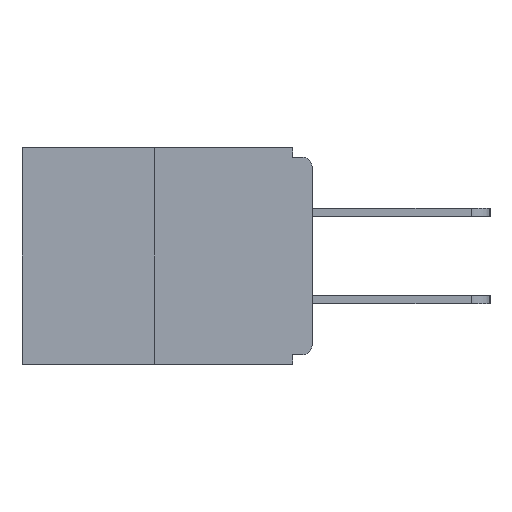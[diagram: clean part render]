
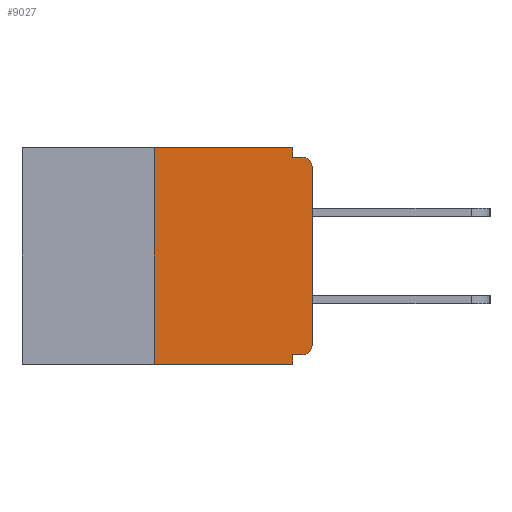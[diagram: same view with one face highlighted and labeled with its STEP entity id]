
A CAD part, left-side view. The second image highlights one B-rep face of the part: STEP entity #9027.
In plain terms, the highlighted planar face has unit normal (-1, 0, 0).
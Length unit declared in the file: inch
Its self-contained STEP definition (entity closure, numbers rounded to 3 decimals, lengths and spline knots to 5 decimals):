
#261 = CARTESIAN_POINT ( 'NONE',  ( 0., 0., -0.313 ) ) ;
#437 = ORIENTED_EDGE ( 'NONE', *, *, #20710, .F. ) ;
#1128 = DIRECTION ( 'NONE',  ( 0., 0., -1. ) ) ;
#1268 = DIRECTION ( 'NONE',  ( 0., 0., 1. ) ) ;
#1305 = CARTESIAN_POINT ( 'NONE',  ( 0., 0.031, -0.015 ) ) ;
#1524 = CARTESIAN_POINT ( 'NONE',  ( 0., 0., 0. ) ) ;
#2679 = LINE ( 'NONE', #7748, #10173 ) ;
#2927 = AXIS2_PLACEMENT_3D ( 'NONE', #16775, #23106, #1128 ) ;
#3027 = LINE ( 'NONE', #24769, #15173 ) ;
#3194 = ORIENTED_EDGE ( 'NONE', *, *, #22684, .T. ) ;
#3237 = DIRECTION ( 'NONE',  ( 0., -1., 0. ) ) ;
#3621 = CARTESIAN_POINT ( 'NONE',  ( 0., 0.031, 0. ) ) ;
#3947 = FACE_OUTER_BOUND ( 'NONE', #13196, .T. ) ;
#4283 = LINE ( 'NONE', #8755, #5694 ) ;
#4379 = AXIS2_PLACEMENT_3D ( 'NONE', #14721, #16600, #27711 ) ;
#4413 = EDGE_CURVE ( 'NONE', #26458, #11795, #27263, .T. ) ;
#4925 = CARTESIAN_POINT ( 'NONE',  ( 0., 0., -0.03 ) ) ;
#5112 = CARTESIAN_POINT ( 'NONE',  ( 0., 0.031, -0.328 ) ) ;
#5694 = VECTOR ( 'NONE', #12999, 39.37008 ) ;
#6394 = ORIENTED_EDGE ( 'NONE', *, *, #4413, .T. ) ;
#6710 = EDGE_CURVE ( 'NONE', #12282, #9344, #3027, .T. ) ;
#7748 = CARTESIAN_POINT ( 'NONE',  ( 0., 0.031, -0.343 ) ) ;
#8276 = CARTESIAN_POINT ( 'NONE',  ( 0., 0.015, -0.328 ) ) ;
#8527 = DIRECTION ( 'NONE',  ( 0., 0., -1. ) ) ;
#8755 = CARTESIAN_POINT ( 'NONE',  ( 0., 0., -0.328 ) ) ;
#9027 = ADVANCED_FACE ( 'NONE', ( #3947 ), #27689, .F. ) ;
#9151 = CARTESIAN_POINT ( 'NONE',  ( 0., 0.25, -0.343 ) ) ;
#9344 = VERTEX_POINT ( 'NONE', #3621 ) ;
#9543 = DIRECTION ( 'NONE',  ( 0., -1., 0. ) ) ;
#10173 = VECTOR ( 'NONE', #20523, 39.37008 ) ;
#10186 = VERTEX_POINT ( 'NONE', #8276 ) ;
#10757 = DIRECTION ( 'NONE',  ( 0., 0., -1. ) ) ;
#10829 = VERTEX_POINT ( 'NONE', #261 ) ;
#10928 = EDGE_CURVE ( 'NONE', #23420, #19906, #15781, .T. ) ;
#11022 = CARTESIAN_POINT ( 'NONE',  ( 0., 0.015, -0.015 ) ) ;
#11795 = VERTEX_POINT ( 'NONE', #24815 ) ;
#11816 = ORIENTED_EDGE ( 'NONE', *, *, #22833, .T. ) ;
#11881 = CARTESIAN_POINT ( 'NONE',  ( 0., 0., -0.015 ) ) ;
#12282 = VERTEX_POINT ( 'NONE', #23031 ) ;
#12361 = ORIENTED_EDGE ( 'NONE', *, *, #6710, .F. ) ;
#12999 = DIRECTION ( 'NONE',  ( 0., 1., 0. ) ) ;
#13196 = EDGE_LOOP ( 'NONE', ( #12361, #14241, #6394, #20639, #13666, #11816, #3194, #20376, #25923, #437 ) ) ;
#13666 = ORIENTED_EDGE ( 'NONE', *, *, #19417, .F. ) ;
#14241 = ORIENTED_EDGE ( 'NONE', *, *, #21060, .F. ) ;
#14721 = CARTESIAN_POINT ( 'NONE',  ( 0., 0.015, -0.313 ) ) ;
#15173 = VECTOR ( 'NONE', #9543, 39.37008 ) ;
#15293 = VECTOR ( 'NONE', #20258, 39.37008 ) ;
#15540 = CARTESIAN_POINT ( 'NONE',  ( 0., 0.46, 0. ) ) ;
#15781 = LINE ( 'NONE', #11881, #15293 ) ;
#15897 = EDGE_CURVE ( 'NONE', #18641, #19906, #17770, .T. ) ;
#16509 = VERTEX_POINT ( 'NONE', #5112 ) ;
#16600 = DIRECTION ( 'NONE',  ( -1., 0., 0. ) ) ;
#16775 = CARTESIAN_POINT ( 'NONE',  ( 0., 0.015, -0.03 ) ) ;
#17770 = CIRCLE ( 'NONE', #2927, 0.015 ) ;
#18637 = VECTOR ( 'NONE', #8527, 39.37008 ) ;
#18641 = VERTEX_POINT ( 'NONE', #4925 ) ;
#19138 = VECTOR ( 'NONE', #1268, 39.37008 ) ;
#19417 = EDGE_CURVE ( 'NONE', #10186, #16509, #4283, .T. ) ;
#19906 = VERTEX_POINT ( 'NONE', #11022 ) ;
#20258 = DIRECTION ( 'NONE',  ( 0., -1., 0. ) ) ;
#20376 = ORIENTED_EDGE ( 'NONE', *, *, #15897, .T. ) ;
#20523 = DIRECTION ( 'NONE',  ( 0., 0., -1. ) ) ;
#20639 = ORIENTED_EDGE ( 'NONE', *, *, #23758, .F. ) ;
#20710 = EDGE_CURVE ( 'NONE', #9344, #23420, #23997, .T. ) ;
#21060 = EDGE_CURVE ( 'NONE', #26458, #12282, #23120, .T. ) ;
#21510 = LINE ( 'NONE', #1524, #22396 ) ;
#21942 = CIRCLE ( 'NONE', #4379, 0.015 ) ;
#22152 = DIRECTION ( 'NONE',  ( 1., 0., 0. ) ) ;
#22396 = VECTOR ( 'NONE', #25976, 39.37008 ) ;
#22684 = EDGE_CURVE ( 'NONE', #10829, #18641, #21510, .T. ) ;
#22833 = EDGE_CURVE ( 'NONE', #10186, #10829, #21942, .T. ) ;
#22939 = CARTESIAN_POINT ( 'NONE',  ( 0., 0.46, -0.343 ) ) ;
#23031 = CARTESIAN_POINT ( 'NONE',  ( 0., 0.25, 0. ) ) ;
#23106 = DIRECTION ( 'NONE',  ( -1., 0., 0. ) ) ;
#23120 = LINE ( 'NONE', #27614, #19138 ) ;
#23420 = VERTEX_POINT ( 'NONE', #1305 ) ;
#23758 = EDGE_CURVE ( 'NONE', #16509, #11795, #2679, .T. ) ;
#23997 = LINE ( 'NONE', #28371, #18637 ) ;
#24769 = CARTESIAN_POINT ( 'NONE',  ( 0., 0.46, 0. ) ) ;
#24815 = CARTESIAN_POINT ( 'NONE',  ( 0., 0.031, -0.343 ) ) ;
#25923 = ORIENTED_EDGE ( 'NONE', *, *, #10928, .F. ) ;
#25976 = DIRECTION ( 'NONE',  ( 0., 0., 1. ) ) ;
#26234 = VECTOR ( 'NONE', #3237, 39.37008 ) ;
#26458 = VERTEX_POINT ( 'NONE', #9151 ) ;
#26816 = AXIS2_PLACEMENT_3D ( 'NONE', #15540, #22152, #10757 ) ;
#27263 = LINE ( 'NONE', #22939, #26234 ) ;
#27614 = CARTESIAN_POINT ( 'NONE',  ( 0., 0.25, 0. ) ) ;
#27689 = PLANE ( 'NONE',  #26816 ) ;
#27711 = DIRECTION ( 'NONE',  ( 0., 0., -1. ) ) ;
#28371 = CARTESIAN_POINT ( 'NONE',  ( 0., 0.031, 0. ) ) ;
